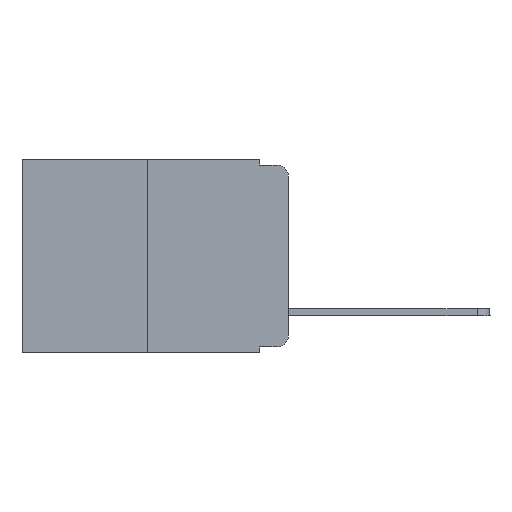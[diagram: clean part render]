
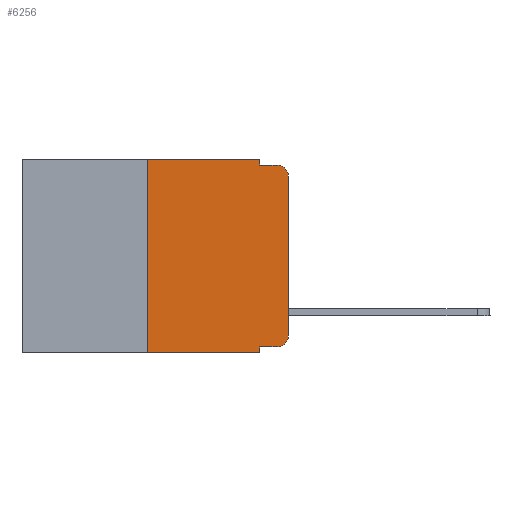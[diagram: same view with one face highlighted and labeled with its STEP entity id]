
A CAD part, left-side view. The second image highlights one B-rep face of the part: STEP entity #6256.
In plain terms, the highlighted planar face has unit normal (-1, 0, 0).
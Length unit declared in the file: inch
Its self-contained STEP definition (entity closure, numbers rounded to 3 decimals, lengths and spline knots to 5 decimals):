
#232 = FACE_OUTER_BOUND ( 'NONE', #6007, .T. ) ;
#630 = CARTESIAN_POINT ( 'NONE',  ( 0., 0.051, 0. ) ) ;
#635 = CARTESIAN_POINT ( 'NONE',  ( 0., 0.051, 0. ) ) ;
#707 = EDGE_CURVE ( 'NONE', #19478, #2010, #7550, .T. ) ;
#824 = AXIS2_PLACEMENT_3D ( 'NONE', #14971, #5891, #4411 ) ;
#1348 = CARTESIAN_POINT ( 'NONE',  ( 0., 0.25, -0.343 ) ) ;
#1542 = CARTESIAN_POINT ( 'NONE',  ( 0., 0., -0.313 ) ) ;
#1674 = CARTESIAN_POINT ( 'NONE',  ( 0., 0.051, -0.333 ) ) ;
#2003 = CARTESIAN_POINT ( 'NONE',  ( 0., 0.25, 0. ) ) ;
#2010 = VERTEX_POINT ( 'NONE', #14284 ) ;
#2092 = DIRECTION ( 'NONE',  ( 0., 0., -1. ) ) ;
#2880 = CARTESIAN_POINT ( 'NONE',  ( 0., 0.473, -0.343 ) ) ;
#3039 = CARTESIAN_POINT ( 'NONE',  ( 0., 0.473, 0. ) ) ;
#3551 = VECTOR ( 'NONE', #13379, 39.37008 ) ;
#3801 = VECTOR ( 'NONE', #13265, 39.37008 ) ;
#4039 = LINE ( 'NONE', #12399, #11317 ) ;
#4041 = ORIENTED_EDGE ( 'NONE', *, *, #14288, .F. ) ;
#4300 = CIRCLE ( 'NONE', #824, 0.02 ) ;
#4305 = PLANE ( 'NONE',  #17054 ) ;
#4384 = CARTESIAN_POINT ( 'NONE',  ( 0., 0.473, 0. ) ) ;
#4411 = DIRECTION ( 'NONE',  ( 0., 0., -1. ) ) ;
#4495 = LINE ( 'NONE', #10190, #3801 ) ;
#4717 = VERTEX_POINT ( 'NONE', #11086 ) ;
#4778 = ORIENTED_EDGE ( 'NONE', *, *, #16276, .F. ) ;
#4867 = VECTOR ( 'NONE', #6009, 39.37008 ) ;
#5290 = ORIENTED_EDGE ( 'NONE', *, *, #9088, .T. ) ;
#5354 = LINE ( 'NONE', #1674, #17141 ) ;
#5430 = VERTEX_POINT ( 'NONE', #630 ) ;
#5519 = DIRECTION ( 'NONE',  ( 0., 0., -1. ) ) ;
#5867 = VERTEX_POINT ( 'NONE', #6100 ) ;
#5891 = DIRECTION ( 'NONE',  ( -1., 0., 0. ) ) ;
#6007 = EDGE_LOOP ( 'NONE', ( #18973, #12476, #17891, #7138, #16524, #4778, #13256, #4041, #5290, #18284 ) ) ;
#6009 = DIRECTION ( 'NONE',  ( 0., -1., 0. ) ) ;
#6080 = VERTEX_POINT ( 'NONE', #18655 ) ;
#6100 = CARTESIAN_POINT ( 'NONE',  ( 0., 0.02, -0.01 ) ) ;
#6256 = ADVANCED_FACE ( 'NONE', ( #232 ), #4305, .F. ) ;
#6731 = LINE ( 'NONE', #2003, #13706 ) ;
#6908 = CARTESIAN_POINT ( 'NONE',  ( 0., 0.051, -0.333 ) ) ;
#7138 = ORIENTED_EDGE ( 'NONE', *, *, #14452, .F. ) ;
#7550 = LINE ( 'NONE', #8875, #3551 ) ;
#7804 = DIRECTION ( 'NONE',  ( 0., -1., 0. ) ) ;
#7924 = LINE ( 'NONE', #2880, #4867 ) ;
#8261 = EDGE_CURVE ( 'NONE', #8832, #5430, #19020, .T. ) ;
#8832 = VERTEX_POINT ( 'NONE', #8897 ) ;
#8875 = CARTESIAN_POINT ( 'NONE',  ( 0., 0., 0. ) ) ;
#8897 = CARTESIAN_POINT ( 'NONE',  ( 0., 0.25, 0. ) ) ;
#9088 = EDGE_CURVE ( 'NONE', #15558, #6080, #5354, .T. ) ;
#10190 = CARTESIAN_POINT ( 'NONE',  ( 0., 0.051, 0. ) ) ;
#10306 = DIRECTION ( 'NONE',  ( 1., 0., 0. ) ) ;
#10785 = DIRECTION ( 'NONE',  ( 0., -1., 0. ) ) ;
#10973 = EDGE_CURVE ( 'NONE', #12124, #4717, #7924, .T. ) ;
#11086 = CARTESIAN_POINT ( 'NONE',  ( 0., 0.051, -0.343 ) ) ;
#11317 = VECTOR ( 'NONE', #10785, 39.37008 ) ;
#12124 = VERTEX_POINT ( 'NONE', #1348 ) ;
#12399 = CARTESIAN_POINT ( 'NONE',  ( 0., 0.051, -0.01 ) ) ;
#12476 = ORIENTED_EDGE ( 'NONE', *, *, #14304, .T. ) ;
#13256 = ORIENTED_EDGE ( 'NONE', *, *, #10973, .T. ) ;
#13265 = DIRECTION ( 'NONE',  ( 0., 0., -1. ) ) ;
#13379 = DIRECTION ( 'NONE',  ( 0., 0., 1. ) ) ;
#13449 = VECTOR ( 'NONE', #2092, 39.37008 ) ;
#13453 = EDGE_CURVE ( 'NONE', #6080, #19478, #4300, .T. ) ;
#13577 = DIRECTION ( 'NONE',  ( 0., 0., -1. ) ) ;
#13706 = VECTOR ( 'NONE', #13994, 39.37008 ) ;
#13994 = DIRECTION ( 'NONE',  ( 0., 0., 1. ) ) ;
#14104 = EDGE_CURVE ( 'NONE', #19018, #5867, #4039, .T. ) ;
#14284 = CARTESIAN_POINT ( 'NONE',  ( 0., 0., -0.03 ) ) ;
#14288 = EDGE_CURVE ( 'NONE', #15558, #4717, #17477, .T. ) ;
#14304 = EDGE_CURVE ( 'NONE', #2010, #5867, #17256, .T. ) ;
#14452 = EDGE_CURVE ( 'NONE', #5430, #19018, #4495, .T. ) ;
#14971 = CARTESIAN_POINT ( 'NONE',  ( 0., 0.02, -0.313 ) ) ;
#15034 = VECTOR ( 'NONE', #15130, 39.37008 ) ;
#15130 = DIRECTION ( 'NONE',  ( 0., -1., 0. ) ) ;
#15558 = VERTEX_POINT ( 'NONE', #6908 ) ;
#16276 = EDGE_CURVE ( 'NONE', #12124, #8832, #6731, .T. ) ;
#16524 = ORIENTED_EDGE ( 'NONE', *, *, #8261, .F. ) ;
#17054 = AXIS2_PLACEMENT_3D ( 'NONE', #3039, #10306, #13577 ) ;
#17141 = VECTOR ( 'NONE', #7804, 39.37008 ) ;
#17256 = CIRCLE ( 'NONE', #17502, 0.02 ) ;
#17477 = LINE ( 'NONE', #635, #13449 ) ;
#17502 = AXIS2_PLACEMENT_3D ( 'NONE', #17569, #19066, #5519 ) ;
#17569 = CARTESIAN_POINT ( 'NONE',  ( 0., 0.02, -0.03 ) ) ;
#17891 = ORIENTED_EDGE ( 'NONE', *, *, #14104, .F. ) ;
#18284 = ORIENTED_EDGE ( 'NONE', *, *, #13453, .T. ) ;
#18655 = CARTESIAN_POINT ( 'NONE',  ( 0., 0.02, -0.333 ) ) ;
#18680 = CARTESIAN_POINT ( 'NONE',  ( 0., 0.051, -0.01 ) ) ;
#18973 = ORIENTED_EDGE ( 'NONE', *, *, #707, .T. ) ;
#19018 = VERTEX_POINT ( 'NONE', #18680 ) ;
#19020 = LINE ( 'NONE', #4384, #15034 ) ;
#19066 = DIRECTION ( 'NONE',  ( -1., 0., 0. ) ) ;
#19478 = VERTEX_POINT ( 'NONE', #1542 ) ;
